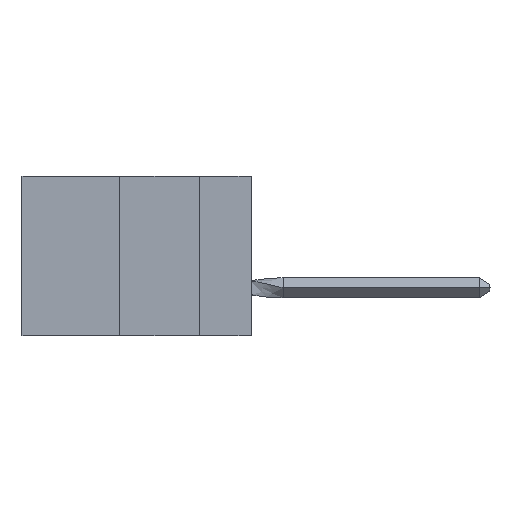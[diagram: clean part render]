
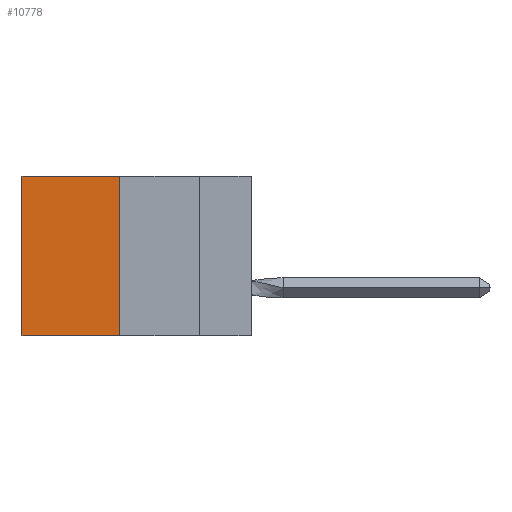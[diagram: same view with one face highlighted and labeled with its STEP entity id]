
A CAD part, left-side view. The second image highlights one B-rep face of the part: STEP entity #10778.
In plain terms, the highlighted planar face has unit normal (-1, 0, 0).
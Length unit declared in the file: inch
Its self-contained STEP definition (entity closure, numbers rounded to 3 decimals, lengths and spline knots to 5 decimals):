
#572 = VECTOR ( 'NONE', #3587, 39.37008 ) ;
#1772 = CARTESIAN_POINT ( 'NONE',  ( 0.305, 0.413, 0. ) ) ;
#2264 = DIRECTION ( 'NONE',  ( 0., 1., 0. ) ) ;
#2328 = DIRECTION ( 'NONE',  ( 0., 1., 0. ) ) ;
#2387 = CARTESIAN_POINT ( 'NONE',  ( 0.305, 0.413, -0.5 ) ) ;
#2908 = ORIENTED_EDGE ( 'NONE', *, *, #13689, .T. ) ;
#2928 = VECTOR ( 'NONE', #2264, 39.37008 ) ;
#3263 = ORIENTED_EDGE ( 'NONE', *, *, #7477, .F. ) ;
#3438 = CARTESIAN_POINT ( 'NONE',  ( 0.305, 0.72, 0. ) ) ;
#3587 = DIRECTION ( 'NONE',  ( 0., 0., -1. ) ) ;
#3661 = LINE ( 'NONE', #4317, #2928 ) ;
#3749 = DIRECTION ( 'NONE',  ( 0., 0., -1. ) ) ;
#3893 = VERTEX_POINT ( 'NONE', #3438 ) ;
#4157 = LINE ( 'NONE', #6997, #572 ) ;
#4317 = CARTESIAN_POINT ( 'NONE',  ( 0.305, 0.413, 0. ) ) ;
#4670 = CARTESIAN_POINT ( 'NONE',  ( 0.305, 0.413, -0.5 ) ) ;
#5061 = EDGE_LOOP ( 'NONE', ( #2908, #10323, #3263, #12336 ) ) ;
#5505 = EDGE_CURVE ( 'NONE', #13445, #13688, #14374, .T. ) ;
#5782 = DIRECTION ( 'NONE',  ( 0., 0., -1. ) ) ;
#6176 = DIRECTION ( 'NONE',  ( 1., 0., 0. ) ) ;
#6417 = FACE_OUTER_BOUND ( 'NONE', #5061, .T. ) ;
#6513 = VERTEX_POINT ( 'NONE', #1772 ) ;
#6683 = AXIS2_PLACEMENT_3D ( 'NONE', #9740, #6176, #3749 ) ;
#6997 = CARTESIAN_POINT ( 'NONE',  ( 0.305, 0.72, -0.5 ) ) ;
#7041 = EDGE_CURVE ( 'NONE', #6513, #3893, #3661, .T. ) ;
#7477 = EDGE_CURVE ( 'NONE', #6513, #13445, #14874, .T. ) ;
#8177 = VECTOR ( 'NONE', #5782, 39.37008 ) ;
#8567 = PLANE ( 'NONE',  #6683 ) ;
#9740 = CARTESIAN_POINT ( 'NONE',  ( 0.305, 0.413, -0.5 ) ) ;
#9998 = CARTESIAN_POINT ( 'NONE',  ( 0.305, 0.413, -0.5 ) ) ;
#10323 = ORIENTED_EDGE ( 'NONE', *, *, #5505, .F. ) ;
#10778 = ADVANCED_FACE ( 'NONE', ( #6417 ), #8567, .F. ) ;
#11473 = VECTOR ( 'NONE', #2328, 39.37008 ) ;
#12336 = ORIENTED_EDGE ( 'NONE', *, *, #7041, .T. ) ;
#12995 = CARTESIAN_POINT ( 'NONE',  ( 0.305, 0.72, -0.5 ) ) ;
#13445 = VERTEX_POINT ( 'NONE', #9998 ) ;
#13688 = VERTEX_POINT ( 'NONE', #12995 ) ;
#13689 = EDGE_CURVE ( 'NONE', #3893, #13688, #4157, .T. ) ;
#14374 = LINE ( 'NONE', #4670, #11473 ) ;
#14874 = LINE ( 'NONE', #2387, #8177 ) ;
